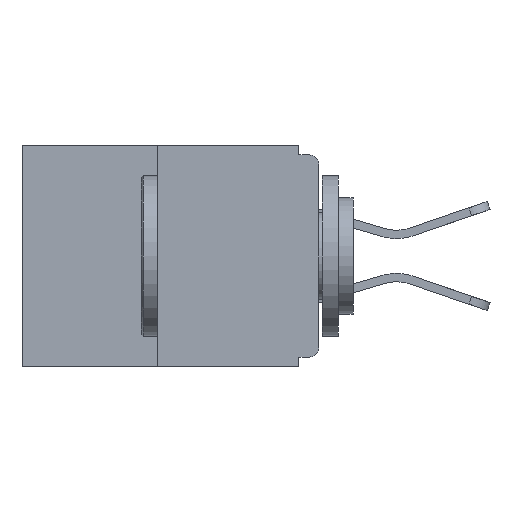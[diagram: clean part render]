
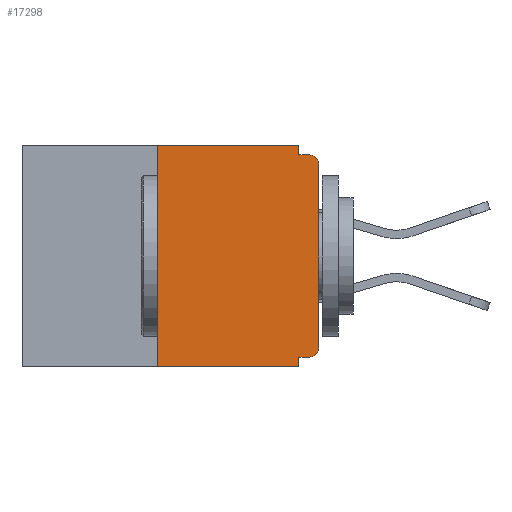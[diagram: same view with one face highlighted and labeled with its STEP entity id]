
A CAD part, left-side view. The second image highlights one B-rep face of the part: STEP entity #17298.
In plain terms, the highlighted planar face has unit normal (-1, 0, 0).
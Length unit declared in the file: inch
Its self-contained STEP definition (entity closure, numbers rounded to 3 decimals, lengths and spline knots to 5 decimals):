
#210 = DIRECTION ( 'NONE',  ( 0., 0., 1. ) ) ;
#653 = VECTOR ( 'NONE', #3241, 39.37008 ) ;
#781 = ORIENTED_EDGE ( 'NONE', *, *, #9179, .F. ) ;
#923 = CARTESIAN_POINT ( 'NONE',  ( 0., 0.015, -0.328 ) ) ;
#936 = LINE ( 'NONE', #12107, #7050 ) ;
#1204 = VERTEX_POINT ( 'NONE', #11589 ) ;
#1345 = AXIS2_PLACEMENT_3D ( 'NONE', #9296, #9538, #10891 ) ;
#1389 = CARTESIAN_POINT ( 'NONE',  ( 0., 0.015, -0.015 ) ) ;
#1614 = DIRECTION ( 'NONE',  ( 0., 0., 1. ) ) ;
#1709 = DIRECTION ( 'NONE',  ( 0., 1., 0. ) ) ;
#1786 = DIRECTION ( 'NONE',  ( 0., -1., 0. ) ) ;
#1825 = EDGE_CURVE ( 'NONE', #3878, #3860, #14484, .T. ) ;
#1911 = ORIENTED_EDGE ( 'NONE', *, *, #11399, .T. ) ;
#2056 = LINE ( 'NONE', #4768, #9446 ) ;
#2168 = VERTEX_POINT ( 'NONE', #10740 ) ;
#2247 = ORIENTED_EDGE ( 'NONE', *, *, #4383, .F. ) ;
#2310 = ORIENTED_EDGE ( 'NONE', *, *, #6938, .T. ) ;
#2331 = ORIENTED_EDGE ( 'NONE', *, *, #16512, .T. ) ;
#2399 = EDGE_CURVE ( 'NONE', #6419, #1204, #3777, .T. ) ;
#3118 = CARTESIAN_POINT ( 'NONE',  ( 0., 0., 0. ) ) ;
#3241 = DIRECTION ( 'NONE',  ( 0., 0., -1. ) ) ;
#3777 = CIRCLE ( 'NONE', #1345, 0.015 ) ;
#3860 = VERTEX_POINT ( 'NONE', #1389 ) ;
#3878 = VERTEX_POINT ( 'NONE', #8254 ) ;
#4340 = CARTESIAN_POINT ( 'NONE',  ( 0., 0., -0.015 ) ) ;
#4383 = EDGE_CURVE ( 'NONE', #8869, #3878, #936, .T. ) ;
#4768 = CARTESIAN_POINT ( 'NONE',  ( 0., 0.46, -0.343 ) ) ;
#5022 = VECTOR ( 'NONE', #1786, 39.37008 ) ;
#5119 = LINE ( 'NONE', #14162, #5547 ) ;
#5411 = VERTEX_POINT ( 'NONE', #7118 ) ;
#5538 = CARTESIAN_POINT ( 'NONE',  ( 0., 0.031, 0. ) ) ;
#5547 = VECTOR ( 'NONE', #13005, 39.37008 ) ;
#6035 = VERTEX_POINT ( 'NONE', #14026 ) ;
#6050 = CARTESIAN_POINT ( 'NONE',  ( 0., 0.015, -0.03 ) ) ;
#6053 = DIRECTION ( 'NONE',  ( 0., 0., -1. ) ) ;
#6114 = PLANE ( 'NONE',  #8907 ) ;
#6353 = LINE ( 'NONE', #11273, #653 ) ;
#6366 = LINE ( 'NONE', #7085, #8065 ) ;
#6419 = VERTEX_POINT ( 'NONE', #923 ) ;
#6489 = VERTEX_POINT ( 'NONE', #16822 ) ;
#6912 = CARTESIAN_POINT ( 'NONE',  ( 0., 0.25, 0. ) ) ;
#6938 = EDGE_CURVE ( 'NONE', #6489, #2168, #2056, .T. ) ;
#7050 = VECTOR ( 'NONE', #13357, 39.37008 ) ;
#7085 = CARTESIAN_POINT ( 'NONE',  ( 0., 0., -0.328 ) ) ;
#7118 = CARTESIAN_POINT ( 'NONE',  ( 0., 0., -0.03 ) ) ;
#7289 = VERTEX_POINT ( 'NONE', #12145 ) ;
#7905 = EDGE_CURVE ( 'NONE', #7289, #8869, #5119, .T. ) ;
#8065 = VECTOR ( 'NONE', #1709, 39.37008 ) ;
#8152 = EDGE_CURVE ( 'NONE', #6489, #7289, #8505, .T. ) ;
#8213 = EDGE_LOOP ( 'NONE', ( #12029, #10460, #2310, #781, #16142, #12683, #2331, #1911, #13427, #2247 ) ) ;
#8254 = CARTESIAN_POINT ( 'NONE',  ( 0., 0.031, -0.015 ) ) ;
#8286 = VECTOR ( 'NONE', #210, 39.37008 ) ;
#8505 = LINE ( 'NONE', #6912, #8286 ) ;
#8712 = EDGE_CURVE ( 'NONE', #6419, #6035, #6366, .T. ) ;
#8768 = DIRECTION ( 'NONE',  ( 0., 0., -1. ) ) ;
#8869 = VERTEX_POINT ( 'NONE', #5538 ) ;
#8907 = AXIS2_PLACEMENT_3D ( 'NONE', #16881, #11378, #6053 ) ;
#9179 = EDGE_CURVE ( 'NONE', #6035, #2168, #6353, .T. ) ;
#9296 = CARTESIAN_POINT ( 'NONE',  ( 0., 0.015, -0.313 ) ) ;
#9446 = VECTOR ( 'NONE', #14188, 39.37008 ) ;
#9538 = DIRECTION ( 'NONE',  ( -1., 0., 0. ) ) ;
#10460 = ORIENTED_EDGE ( 'NONE', *, *, #8152, .F. ) ;
#10706 = LINE ( 'NONE', #3118, #12167 ) ;
#10740 = CARTESIAN_POINT ( 'NONE',  ( 0., 0.031, -0.343 ) ) ;
#10891 = DIRECTION ( 'NONE',  ( 0., 0., -1. ) ) ;
#11197 = AXIS2_PLACEMENT_3D ( 'NONE', #6050, #15436, #8768 ) ;
#11273 = CARTESIAN_POINT ( 'NONE',  ( 0., 0.031, -0.343 ) ) ;
#11378 = DIRECTION ( 'NONE',  ( 1., 0., 0. ) ) ;
#11399 = EDGE_CURVE ( 'NONE', #5411, #3860, #12206, .T. ) ;
#11589 = CARTESIAN_POINT ( 'NONE',  ( 0., 0., -0.313 ) ) ;
#12029 = ORIENTED_EDGE ( 'NONE', *, *, #7905, .F. ) ;
#12107 = CARTESIAN_POINT ( 'NONE',  ( 0., 0.031, 0. ) ) ;
#12145 = CARTESIAN_POINT ( 'NONE',  ( 0., 0.25, 0. ) ) ;
#12167 = VECTOR ( 'NONE', #1614, 39.37008 ) ;
#12206 = CIRCLE ( 'NONE', #11197, 0.015 ) ;
#12683 = ORIENTED_EDGE ( 'NONE', *, *, #2399, .T. ) ;
#13005 = DIRECTION ( 'NONE',  ( 0., -1., 0. ) ) ;
#13357 = DIRECTION ( 'NONE',  ( 0., 0., -1. ) ) ;
#13427 = ORIENTED_EDGE ( 'NONE', *, *, #1825, .F. ) ;
#14026 = CARTESIAN_POINT ( 'NONE',  ( 0., 0.031, -0.328 ) ) ;
#14162 = CARTESIAN_POINT ( 'NONE',  ( 0., 0.46, 0. ) ) ;
#14188 = DIRECTION ( 'NONE',  ( 0., -1., 0. ) ) ;
#14484 = LINE ( 'NONE', #4340, #5022 ) ;
#15436 = DIRECTION ( 'NONE',  ( -1., 0., 0. ) ) ;
#15892 = FACE_OUTER_BOUND ( 'NONE', #8213, .T. ) ;
#16142 = ORIENTED_EDGE ( 'NONE', *, *, #8712, .F. ) ;
#16512 = EDGE_CURVE ( 'NONE', #1204, #5411, #10706, .T. ) ;
#16822 = CARTESIAN_POINT ( 'NONE',  ( 0., 0.25, -0.343 ) ) ;
#16881 = CARTESIAN_POINT ( 'NONE',  ( 0., 0.46, 0. ) ) ;
#17298 = ADVANCED_FACE ( 'NONE', ( #15892 ), #6114, .F. ) ;
